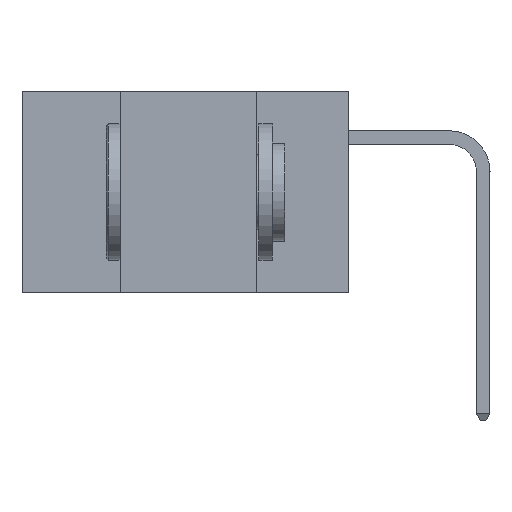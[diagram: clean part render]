
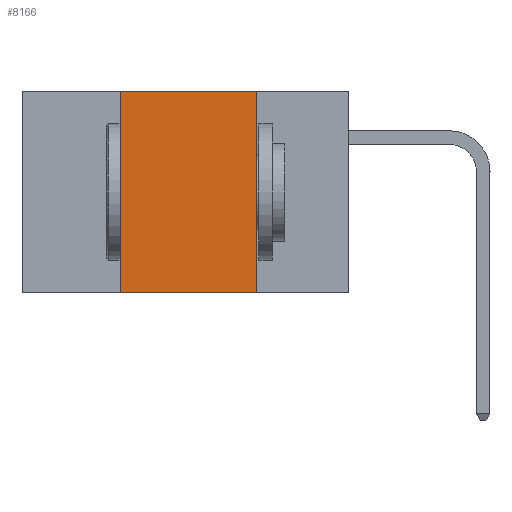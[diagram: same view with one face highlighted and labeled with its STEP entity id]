
A CAD part, left-side view. The second image highlights one B-rep face of the part: STEP entity #8166.
In plain terms, the highlighted planar face has unit normal (-1, 0, 0).
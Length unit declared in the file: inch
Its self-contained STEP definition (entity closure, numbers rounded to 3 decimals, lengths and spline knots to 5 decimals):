
#236 = LINE ( 'NONE', #21168, #10064 ) ;
#1216 = DIRECTION ( 'NONE',  ( 0., 0., -1. ) ) ;
#1483 = ORIENTED_EDGE ( 'NONE', *, *, #34466, .T. ) ;
#1756 = DIRECTION ( 'NONE',  ( 0., -1., 0. ) ) ;
#3241 = DIRECTION ( 'NONE',  ( 0., -1., 0. ) ) ;
#5438 = CARTESIAN_POINT ( 'NONE',  ( 0., 0.17, -0.37 ) ) ;
#6466 = PLANE ( 'NONE',  #9127 ) ;
#6601 = CARTESIAN_POINT ( 'NONE',  ( 0., 0.6, 0. ) ) ;
#6682 = VERTEX_POINT ( 'NONE', #5438 ) ;
#8166 = ADVANCED_FACE ( 'NONE', ( #32596 ), #6466, .F. ) ;
#9127 = AXIS2_PLACEMENT_3D ( 'NONE', #6601, #36526, #16723 ) ;
#9239 = ORIENTED_EDGE ( 'NONE', *, *, #26963, .F. ) ;
#10064 = VECTOR ( 'NONE', #1216, 39.37008 ) ;
#14214 = DIRECTION ( 'NONE',  ( 0., 0., 1. ) ) ;
#16719 = VERTEX_POINT ( 'NONE', #36763 ) ;
#16723 = DIRECTION ( 'NONE',  ( 0., 0., -1. ) ) ;
#17072 = VERTEX_POINT ( 'NONE', #29235 ) ;
#19410 = LINE ( 'NONE', #34053, #35980 ) ;
#19815 = EDGE_CURVE ( 'NONE', #17072, #24861, #42831, .T. ) ;
#21168 = CARTESIAN_POINT ( 'NONE',  ( 0., 0.17, 0. ) ) ;
#21771 = EDGE_CURVE ( 'NONE', #16719, #17072, #19410, .T. ) ;
#23230 = CARTESIAN_POINT ( 'NONE',  ( 0., 0.6, -0.37 ) ) ;
#23388 = CARTESIAN_POINT ( 'NONE',  ( 0., 0.17, 0. ) ) ;
#24861 = VERTEX_POINT ( 'NONE', #23388 ) ;
#25277 = VECTOR ( 'NONE', #1756, 39.37008 ) ;
#25598 = LINE ( 'NONE', #23230, #33309 ) ;
#25958 = ORIENTED_EDGE ( 'NONE', *, *, #21771, .F. ) ;
#26963 = EDGE_CURVE ( 'NONE', #24861, #6682, #236, .T. ) ;
#28339 = CARTESIAN_POINT ( 'NONE',  ( 0., 0.6, 0. ) ) ;
#29235 = CARTESIAN_POINT ( 'NONE',  ( 0., 0.42, 0. ) ) ;
#31980 = EDGE_LOOP ( 'NONE', ( #9239, #33273, #25958, #1483 ) ) ;
#32596 = FACE_OUTER_BOUND ( 'NONE', #31980, .T. ) ;
#33273 = ORIENTED_EDGE ( 'NONE', *, *, #19815, .F. ) ;
#33309 = VECTOR ( 'NONE', #3241, 39.37008 ) ;
#34053 = CARTESIAN_POINT ( 'NONE',  ( 0., 0.42, 0. ) ) ;
#34466 = EDGE_CURVE ( 'NONE', #16719, #6682, #25598, .T. ) ;
#35980 = VECTOR ( 'NONE', #14214, 39.37008 ) ;
#36526 = DIRECTION ( 'NONE',  ( 1., 0., 0. ) ) ;
#36763 = CARTESIAN_POINT ( 'NONE',  ( 0., 0.42, -0.37 ) ) ;
#42831 = LINE ( 'NONE', #28339, #25277 ) ;
